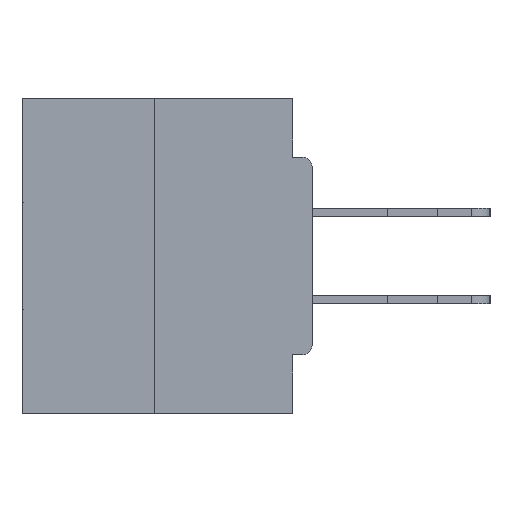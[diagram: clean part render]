
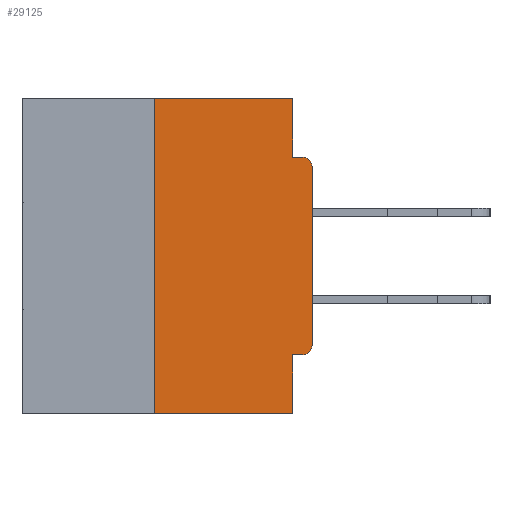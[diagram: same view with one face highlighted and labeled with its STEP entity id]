
A CAD part, left-side view. The second image highlights one B-rep face of the part: STEP entity #29125.
In plain terms, the highlighted planar face has unit normal (-1, 0, 0).
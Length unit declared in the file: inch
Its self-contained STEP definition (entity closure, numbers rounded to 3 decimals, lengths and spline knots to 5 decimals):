
#60 = FACE_OUTER_BOUND ( 'NONE', #37630, .T. ) ;
#216 = LINE ( 'NONE', #25273, #21991 ) ;
#320 = CARTESIAN_POINT ( 'NONE',  ( 0., 0.031, -0.0935 ) ) ;
#460 = LINE ( 'NONE', #20811, #8720 ) ;
#1136 = ORIENTED_EDGE ( 'NONE', *, *, #35528, .F. ) ;
#1139 = CARTESIAN_POINT ( 'NONE',  ( 0., 0.015, -0.3915 ) ) ;
#1273 = VERTEX_POINT ( 'NONE', #28027 ) ;
#1526 = DIRECTION ( 'NONE',  ( -1., 0., 0. ) ) ;
#1908 = VECTOR ( 'NONE', #13959, 39.37008 ) ;
#2796 = ORIENTED_EDGE ( 'NONE', *, *, #16076, .T. ) ;
#4388 = DIRECTION ( 'NONE',  ( -1., 0., 0. ) ) ;
#4531 = VERTEX_POINT ( 'NONE', #16927 ) ;
#6098 = EDGE_CURVE ( 'NONE', #33312, #29081, #25740, .T. ) ;
#6262 = VERTEX_POINT ( 'NONE', #32265 ) ;
#6404 = LINE ( 'NONE', #22757, #21874 ) ;
#6712 = CARTESIAN_POINT ( 'NONE',  ( 0., 0., -0.0935 ) ) ;
#6765 = DIRECTION ( 'NONE',  ( 0., 0., 1. ) ) ;
#8246 = DIRECTION ( 'NONE',  ( 0., 0., 1. ) ) ;
#8720 = VECTOR ( 'NONE', #8246, 39.37008 ) ;
#10133 = DIRECTION ( 'NONE',  ( 1., 0., 0. ) ) ;
#10149 = EDGE_CURVE ( 'NONE', #6262, #34055, #11231, .T. ) ;
#10833 = DIRECTION ( 'NONE',  ( 0., 0., -1. ) ) ;
#11231 = CIRCLE ( 'NONE', #33860, 0.015 ) ;
#13803 = ORIENTED_EDGE ( 'NONE', *, *, #10149, .T. ) ;
#13834 = CARTESIAN_POINT ( 'NONE',  ( 0., 0.46, 0. ) ) ;
#13959 = DIRECTION ( 'NONE',  ( 0., -1., 0. ) ) ;
#14048 = VECTOR ( 'NONE', #30986, 39.37008 ) ;
#16076 = EDGE_CURVE ( 'NONE', #35016, #6262, #216, .T. ) ;
#16190 = CARTESIAN_POINT ( 'NONE',  ( 0., 0., -0.3915 ) ) ;
#16927 = CARTESIAN_POINT ( 'NONE',  ( 0., 0.25, -0.5 ) ) ;
#17253 = ORIENTED_EDGE ( 'NONE', *, *, #39185, .F. ) ;
#17579 = ORIENTED_EDGE ( 'NONE', *, *, #25441, .T. ) ;
#18904 = PLANE ( 'NONE',  #20355 ) ;
#19421 = DIRECTION ( 'NONE',  ( 0., 0., -1. ) ) ;
#19816 = DIRECTION ( 'NONE',  ( 0., 0., -1. ) ) ;
#20355 = AXIS2_PLACEMENT_3D ( 'NONE', #25476, #10133, #19816 ) ;
#20586 = ORIENTED_EDGE ( 'NONE', *, *, #26393, .T. ) ;
#20710 = ORIENTED_EDGE ( 'NONE', *, *, #30071, .F. ) ;
#20811 = CARTESIAN_POINT ( 'NONE',  ( 0., 0.25, 0. ) ) ;
#21191 = VERTEX_POINT ( 'NONE', #28769 ) ;
#21843 = CARTESIAN_POINT ( 'NONE',  ( 0., 0.25, 0. ) ) ;
#21874 = VECTOR ( 'NONE', #25844, 39.37008 ) ;
#21910 = VERTEX_POINT ( 'NONE', #35090 ) ;
#21991 = VECTOR ( 'NONE', #6765, 39.37008 ) ;
#22757 = CARTESIAN_POINT ( 'NONE',  ( 0., 0., -0.4065 ) ) ;
#22758 = CARTESIAN_POINT ( 'NONE',  ( 0., 0.015, -0.1085 ) ) ;
#23217 = LINE ( 'NONE', #6712, #14048 ) ;
#24526 = CARTESIAN_POINT ( 'NONE',  ( 0., 0.031, 0. ) ) ;
#24758 = LINE ( 'NONE', #35233, #31044 ) ;
#25273 = CARTESIAN_POINT ( 'NONE',  ( 0., 0., 0. ) ) ;
#25441 = EDGE_CURVE ( 'NONE', #1273, #35016, #35137, .T. ) ;
#25476 = CARTESIAN_POINT ( 'NONE',  ( 0., 0.46, 0. ) ) ;
#25483 = DIRECTION ( 'NONE',  ( 0., -1., 0. ) ) ;
#25740 = LINE ( 'NONE', #29458, #35421 ) ;
#25844 = DIRECTION ( 'NONE',  ( 0., 1., 0. ) ) ;
#26393 = EDGE_CURVE ( 'NONE', #4531, #21191, #27848, .T. ) ;
#26807 = ORIENTED_EDGE ( 'NONE', *, *, #35410, .F. ) ;
#27848 = LINE ( 'NONE', #28874, #34156 ) ;
#28027 = CARTESIAN_POINT ( 'NONE',  ( 0., 0.015, -0.4065 ) ) ;
#28769 = CARTESIAN_POINT ( 'NONE',  ( 0., 0.031, -0.5 ) ) ;
#28874 = CARTESIAN_POINT ( 'NONE',  ( 0., 0.46, -0.5 ) ) ;
#29081 = VERTEX_POINT ( 'NONE', #320 ) ;
#29125 = ADVANCED_FACE ( 'NONE', ( #60 ), #18904, .F. ) ;
#29173 = EDGE_CURVE ( 'NONE', #21910, #21191, #24758, .T. ) ;
#29458 = CARTESIAN_POINT ( 'NONE',  ( 0., 0.031, 0. ) ) ;
#30071 = EDGE_CURVE ( 'NONE', #29081, #34055, #23217, .T. ) ;
#30450 = LINE ( 'NONE', #13834, #1908 ) ;
#30729 = VERTEX_POINT ( 'NONE', #21843 ) ;
#30986 = DIRECTION ( 'NONE',  ( 0., -1., 0. ) ) ;
#30998 = ORIENTED_EDGE ( 'NONE', *, *, #6098, .F. ) ;
#31044 = VECTOR ( 'NONE', #19421, 39.37008 ) ;
#32089 = DIRECTION ( 'NONE',  ( 0., 0., -1. ) ) ;
#32247 = DIRECTION ( 'NONE',  ( 0., 0., -1. ) ) ;
#32265 = CARTESIAN_POINT ( 'NONE',  ( 0., 0., -0.1085 ) ) ;
#33312 = VERTEX_POINT ( 'NONE', #24526 ) ;
#33860 = AXIS2_PLACEMENT_3D ( 'NONE', #22758, #1526, #32089 ) ;
#34055 = VERTEX_POINT ( 'NONE', #38421 ) ;
#34148 = ORIENTED_EDGE ( 'NONE', *, *, #29173, .F. ) ;
#34156 = VECTOR ( 'NONE', #25483, 39.37008 ) ;
#35016 = VERTEX_POINT ( 'NONE', #16190 ) ;
#35090 = CARTESIAN_POINT ( 'NONE',  ( 0., 0.031, -0.4065 ) ) ;
#35137 = CIRCLE ( 'NONE', #37154, 0.015 ) ;
#35233 = CARTESIAN_POINT ( 'NONE',  ( 0., 0.031, -0.5 ) ) ;
#35410 = EDGE_CURVE ( 'NONE', #30729, #33312, #30450, .T. ) ;
#35421 = VECTOR ( 'NONE', #10833, 39.37008 ) ;
#35528 = EDGE_CURVE ( 'NONE', #4531, #30729, #460, .T. ) ;
#37154 = AXIS2_PLACEMENT_3D ( 'NONE', #1139, #4388, #32247 ) ;
#37630 = EDGE_LOOP ( 'NONE', ( #26807, #1136, #20586, #34148, #17253, #17579, #2796, #13803, #20710, #30998 ) ) ;
#38421 = CARTESIAN_POINT ( 'NONE',  ( 0., 0.015, -0.0935 ) ) ;
#39185 = EDGE_CURVE ( 'NONE', #1273, #21910, #6404, .T. ) ;
